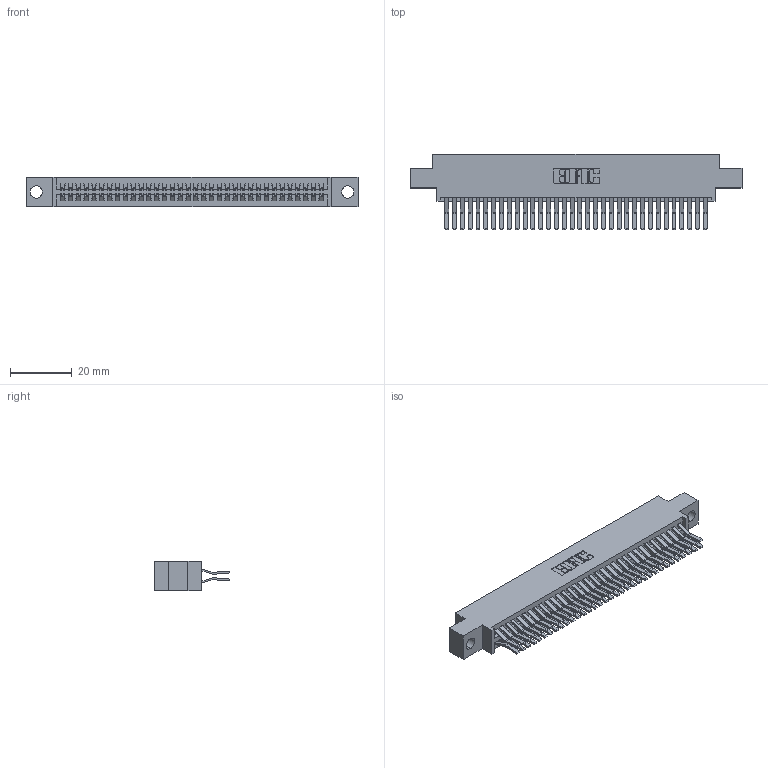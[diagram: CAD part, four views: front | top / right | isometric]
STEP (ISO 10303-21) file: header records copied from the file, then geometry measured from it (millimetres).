
FILE_DESCRIPTION (( 'STEP AP203' ), '1' );
FILE_NAME ('345-068-560-804.STEP', '2021-05-20T08:03:25', ( '' ), ( '' ), 'SwSTEP 2.0', 'SolidWorks 2020', '' );
FILE_SCHEMA (( 'CONFIG_CONTROL_DESIGN' ));
Length unit declared in the file: inch
Products named in the file (3): 345-292-001_560 Tail; 345-068-560-804; 345 Part_0.170 Offset - 0.156 Dia-TI
Assembly tree (69 placements, depth 2):
  345-068-560-804
    345 Part_0.170 Offset - 0.156 Dia-TI
    345-292-001_560 Tail  x68
Bounding box: 107.57 x 24.45 x 9.4 mm (x, y, z)
Volume: 10601.5 mm3; surface area: 16657.2 mm2
Topology: 69 solids, 69 shells, 3680 faces, 10929 edges, 7194 vertices
Faces by surface type: plane 2342, cylinder 1338
Entity records: 28393 total; most frequent: CARTESIAN_POINT 4774, ORIENTED_EDGE 4706, DIRECTION 4221, EDGE_CURVE 2353, VECTOR 2081, LINE 2081, VERTEX_POINT 1566, AXIS2_PLACEMENT_3D 1070
